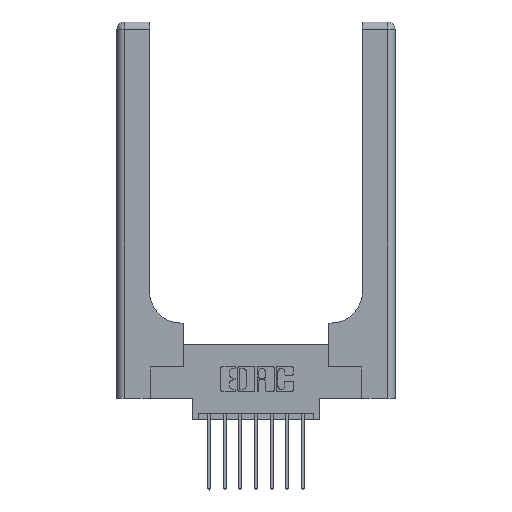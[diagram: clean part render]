
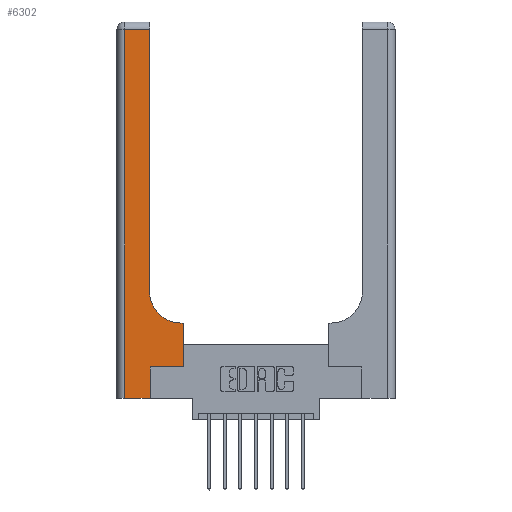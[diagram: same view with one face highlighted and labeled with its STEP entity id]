
A CAD part, top view. The second image highlights one B-rep face of the part: STEP entity #6302.
In plain terms, the highlighted planar face has unit normal (0, 0, 1).
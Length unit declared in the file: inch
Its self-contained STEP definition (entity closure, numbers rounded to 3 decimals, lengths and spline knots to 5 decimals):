
#327 = LINE ( 'NONE', #1338, #12329 ) ;
#588 = LINE ( 'NONE', #4324, #3575 ) ;
#758 = VERTEX_POINT ( 'NONE', #5342 ) ;
#1244 = VERTEX_POINT ( 'NONE', #6373 ) ;
#1338 = CARTESIAN_POINT ( 'NONE',  ( 0.265, 0., 0.37 ) ) ;
#1652 = EDGE_CURVE ( 'NONE', #758, #10777, #4397, .T. ) ;
#1700 = DIRECTION ( 'NONE',  ( 1., 0., 0. ) ) ;
#2211 = CARTESIAN_POINT ( 'NONE',  ( 0.51, 0.85, 0.37 ) ) ;
#2656 = EDGE_CURVE ( 'NONE', #13524, #9949, #327, .T. ) ;
#2955 = AXIS2_PLACEMENT_3D ( 'NONE', #10781, #5162, #13060 ) ;
#3169 = ORIENTED_EDGE ( 'NONE', *, *, #7208, .T. ) ;
#3298 = VERTEX_POINT ( 'NONE', #14083 ) ;
#3366 = DIRECTION ( 'NONE',  ( 1., 0., 0. ) ) ;
#3575 = VECTOR ( 'NONE', #13379, 39.37008 ) ;
#3629 = LINE ( 'NONE', #13462, #8608 ) ;
#3957 = CARTESIAN_POINT ( 'NONE',  ( 0., 0., 0.37 ) ) ;
#3985 = LINE ( 'NONE', #8331, #12282 ) ;
#4018 = PLANE ( 'NONE',  #2955 ) ;
#4095 = CARTESIAN_POINT ( 'NONE',  ( 0.265, 0.25, 0.37 ) ) ;
#4229 = EDGE_CURVE ( 'NONE', #5328, #11626, #3629, .T. ) ;
#4253 = ORIENTED_EDGE ( 'NONE', *, *, #10528, .T. ) ;
#4261 = EDGE_LOOP ( 'NONE', ( #4253, #7649, #7159, #5894, #5857, #9476, #8611, #11527, #3169 ) ) ;
#4324 = CARTESIAN_POINT ( 'NONE',  ( 0.26, 3., 0.37 ) ) ;
#4397 = LINE ( 'NONE', #4954, #13082 ) ;
#4408 = DIRECTION ( 'NONE',  ( 0., -1., 0. ) ) ;
#4764 = CARTESIAN_POINT ( 'NONE',  ( 0., 2.94, 0.37 ) ) ;
#4954 = CARTESIAN_POINT ( 'NONE',  ( 0.26, 0.6, 0.37 ) ) ;
#5162 = DIRECTION ( 'NONE',  ( 0., 0., -1. ) ) ;
#5328 = VERTEX_POINT ( 'NONE', #14527 ) ;
#5342 = CARTESIAN_POINT ( 'NONE',  ( 0.528, 0.6, 0.37 ) ) ;
#5391 = DIRECTION ( 'NONE',  ( 0., 1., 0. ) ) ;
#5541 = VECTOR ( 'NONE', #5391, 39.37008 ) ;
#5704 = LINE ( 'NONE', #4764, #14355 ) ;
#5857 = ORIENTED_EDGE ( 'NONE', *, *, #2656, .T. ) ;
#5894 = ORIENTED_EDGE ( 'NONE', *, *, #9865, .T. ) ;
#6251 = LINE ( 'NONE', #9878, #5541 ) ;
#6302 = ADVANCED_FACE ( 'NONE', ( #12079 ), #4018, .F. ) ;
#6373 = CARTESIAN_POINT ( 'NONE',  ( 0.26, 2.94, 0.37 ) ) ;
#7097 = EDGE_CURVE ( 'NONE', #3298, #758, #6251, .T. ) ;
#7159 = ORIENTED_EDGE ( 'NONE', *, *, #4229, .T. ) ;
#7182 = DIRECTION ( 'NONE',  ( 1., 0., 0. ) ) ;
#7204 = DIRECTION ( 'NONE',  ( -1., 0., 0. ) ) ;
#7208 = EDGE_CURVE ( 'NONE', #10777, #10848, #13131, .T. ) ;
#7386 = EDGE_CURVE ( 'NONE', #1244, #5328, #5704, .T. ) ;
#7649 = ORIENTED_EDGE ( 'NONE', *, *, #7386, .T. ) ;
#7717 = CARTESIAN_POINT ( 'NONE',  ( 0.06, 0., 0.37 ) ) ;
#7905 = CARTESIAN_POINT ( 'NONE',  ( 0.265, 0., 0.37 ) ) ;
#8125 = CARTESIAN_POINT ( 'NONE',  ( 0.51, 0.6, 0.37 ) ) ;
#8266 = CARTESIAN_POINT ( 'NONE',  ( 0.26, 0.85, 0.37 ) ) ;
#8331 = CARTESIAN_POINT ( 'NONE',  ( 0.265, 0.25, 0.37 ) ) ;
#8608 = VECTOR ( 'NONE', #4408, 39.37008 ) ;
#8611 = ORIENTED_EDGE ( 'NONE', *, *, #7097, .T. ) ;
#8639 = EDGE_CURVE ( 'NONE', #9949, #3298, #3985, .T. ) ;
#9230 = DIRECTION ( 'NONE',  ( 0., 1., 0. ) ) ;
#9326 = DIRECTION ( 'NONE',  ( -1., 0., 0. ) ) ;
#9476 = ORIENTED_EDGE ( 'NONE', *, *, #8639, .T. ) ;
#9781 = LINE ( 'NONE', #3957, #12774 ) ;
#9865 = EDGE_CURVE ( 'NONE', #11626, #13524, #9781, .T. ) ;
#9878 = CARTESIAN_POINT ( 'NONE',  ( 0.528, 0.25, 0.37 ) ) ;
#9949 = VERTEX_POINT ( 'NONE', #4095 ) ;
#10114 = DIRECTION ( 'NONE',  ( 0., 0., -1. ) ) ;
#10528 = EDGE_CURVE ( 'NONE', #10848, #1244, #588, .T. ) ;
#10777 = VERTEX_POINT ( 'NONE', #8125 ) ;
#10781 = CARTESIAN_POINT ( 'NONE',  ( 0., 3., 0.37 ) ) ;
#10848 = VERTEX_POINT ( 'NONE', #8266 ) ;
#11527 = ORIENTED_EDGE ( 'NONE', *, *, #1652, .T. ) ;
#11626 = VERTEX_POINT ( 'NONE', #7717 ) ;
#12079 = FACE_OUTER_BOUND ( 'NONE', #4261, .T. ) ;
#12282 = VECTOR ( 'NONE', #7182, 39.37008 ) ;
#12329 = VECTOR ( 'NONE', #9230, 39.37008 ) ;
#12774 = VECTOR ( 'NONE', #1700, 39.37008 ) ;
#13060 = DIRECTION ( 'NONE',  ( -1., 0., 0. ) ) ;
#13082 = VECTOR ( 'NONE', #7204, 39.37008 ) ;
#13131 = CIRCLE ( 'NONE', #13731, 0.25 ) ;
#13379 = DIRECTION ( 'NONE',  ( 0., 1., 0. ) ) ;
#13462 = CARTESIAN_POINT ( 'NONE',  ( 0.06, 3., 0.37 ) ) ;
#13524 = VERTEX_POINT ( 'NONE', #7905 ) ;
#13731 = AXIS2_PLACEMENT_3D ( 'NONE', #2211, #10114, #3366 ) ;
#14083 = CARTESIAN_POINT ( 'NONE',  ( 0.528, 0.25, 0.37 ) ) ;
#14355 = VECTOR ( 'NONE', #9326, 39.37008 ) ;
#14527 = CARTESIAN_POINT ( 'NONE',  ( 0.06, 2.94, 0.37 ) ) ;
